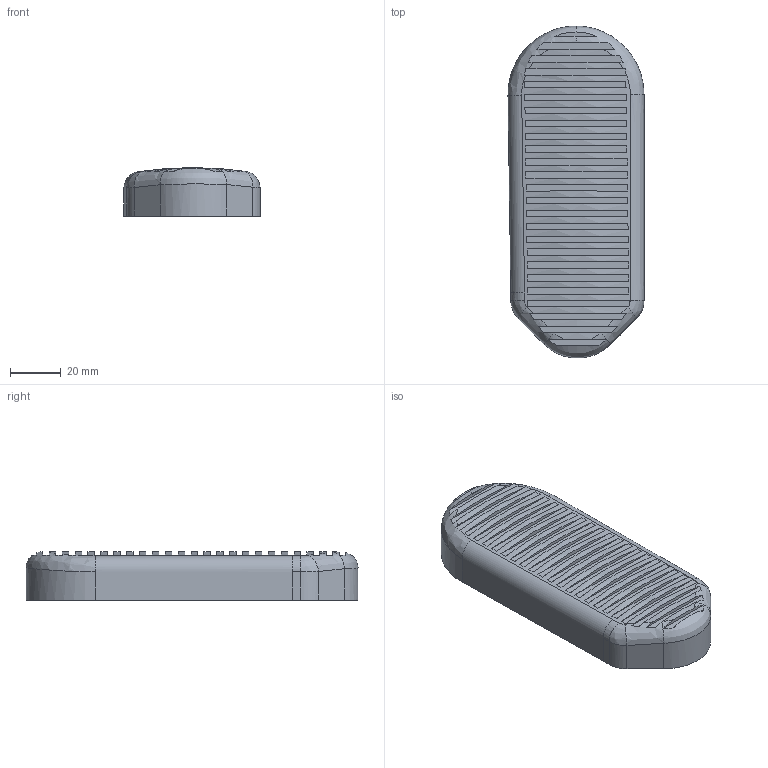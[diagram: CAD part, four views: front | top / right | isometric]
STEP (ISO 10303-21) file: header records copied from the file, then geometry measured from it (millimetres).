
FILE_DESCRIPTION (( 'STEP AP214' ), '1' );
FILE_NAME ('Butt Pad.STEP', '2013-12-11T22:25:11', ( 'elpi' ), ( '' ), 'SwSTEP 2.0', 'SolidWorks 2013', '' );
FILE_SCHEMA (( 'AUTOMOTIVE_DESIGN' ));
Length unit declared in the file: inch
Products named in the file (1): Butt Pad
Bounding box: 53.66 x 130.95 x 19.05 mm (x, y, z)
Volume: 108042.5 mm3; surface area: 19971.2 mm2
Topology: 1 solids, 1 shells, 113 faces, 261 edges, 171 vertices
Faces by surface type: plane 84, bspline 15, cylinder 14
Entity records: 6427 total; most frequent: CARTESIAN_POINT 4125, ORIENTED_EDGE 522, DIRECTION 368, EDGE_CURVE 261, VERTEX_POINT 171, EDGE_LOOP 134, AXIS2_PLACEMENT_3D 127, VECTOR 114
